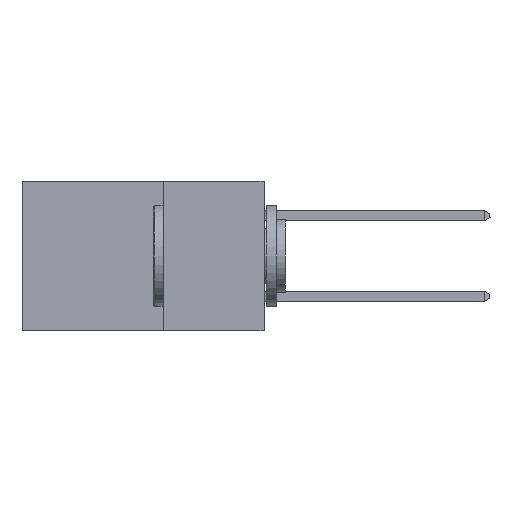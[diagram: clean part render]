
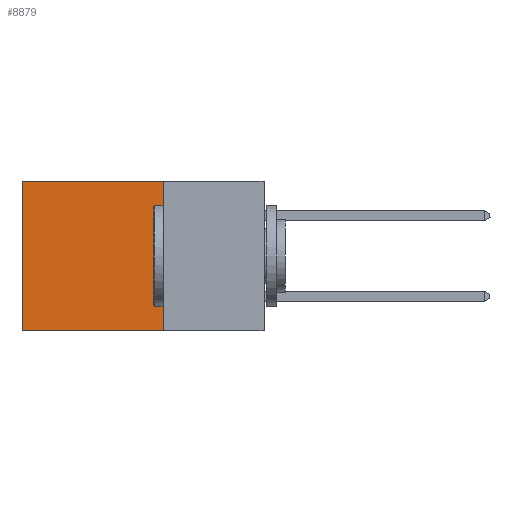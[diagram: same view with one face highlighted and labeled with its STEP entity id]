
A CAD part, left-side view. The second image highlights one B-rep face of the part: STEP entity #8879.
In plain terms, the highlighted planar face has unit normal (-1, 0, 0).
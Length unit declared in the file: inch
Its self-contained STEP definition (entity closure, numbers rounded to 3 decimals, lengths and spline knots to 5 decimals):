
#443 = LINE ( 'NONE', #2643, #15440 ) ;
#2643 = CARTESIAN_POINT ( 'NONE',  ( 0.298, 0.25, 0. ) ) ;
#2981 = CARTESIAN_POINT ( 'NONE',  ( 0.298, 0.25, 0. ) ) ;
#4487 = VERTEX_POINT ( 'NONE', #19841 ) ;
#7111 = AXIS2_PLACEMENT_3D ( 'NONE', #16543, #26297, #11472 ) ;
#8025 = LINE ( 'NONE', #15118, #19415 ) ;
#8879 = ADVANCED_FACE ( 'NONE', ( #30344 ), #21218, .F. ) ;
#10513 = ORIENTED_EDGE ( 'NONE', *, *, #15867, .T. ) ;
#11425 = CARTESIAN_POINT ( 'NONE',  ( 0.298, 0.6, 0. ) ) ;
#11472 = DIRECTION ( 'NONE',  ( 0., 0., -1. ) ) ;
#12732 = DIRECTION ( 'NONE',  ( 0., 0., -1. ) ) ;
#13206 = DIRECTION ( 'NONE',  ( 0., 1., 0. ) ) ;
#14873 = VERTEX_POINT ( 'NONE', #21561 ) ;
#15118 = CARTESIAN_POINT ( 'NONE',  ( 0.298, 0.25, -0.37 ) ) ;
#15440 = VECTOR ( 'NONE', #30175, 39.37008 ) ;
#15867 = EDGE_CURVE ( 'NONE', #4487, #25518, #17449, .T. ) ;
#16543 = CARTESIAN_POINT ( 'NONE',  ( 0.298, 0.25, 0. ) ) ;
#16840 = ORIENTED_EDGE ( 'NONE', *, *, #27438, .T. ) ;
#17449 = LINE ( 'NONE', #11425, #19404 ) ;
#19404 = VECTOR ( 'NONE', #12732, 39.37008 ) ;
#19415 = VECTOR ( 'NONE', #29818, 39.37008 ) ;
#19841 = CARTESIAN_POINT ( 'NONE',  ( 0.298, 0.6, 0. ) ) ;
#20129 = ORIENTED_EDGE ( 'NONE', *, *, #30331, .F. ) ;
#20323 = VECTOR ( 'NONE', #13206, 39.37008 ) ;
#21218 = PLANE ( 'NONE',  #7111 ) ;
#21561 = CARTESIAN_POINT ( 'NONE',  ( 0.298, 0.25, 0. ) ) ;
#22325 = CARTESIAN_POINT ( 'NONE',  ( 0.298, 0.25, -0.37 ) ) ;
#22896 = CARTESIAN_POINT ( 'NONE',  ( 0.298, 0.6, -0.37 ) ) ;
#24707 = ORIENTED_EDGE ( 'NONE', *, *, #28989, .F. ) ;
#25518 = VERTEX_POINT ( 'NONE', #22896 ) ;
#26297 = DIRECTION ( 'NONE',  ( 1., 0., 0. ) ) ;
#26477 = EDGE_LOOP ( 'NONE', ( #10513, #24707, #20129, #16840 ) ) ;
#26702 = VERTEX_POINT ( 'NONE', #22325 ) ;
#27438 = EDGE_CURVE ( 'NONE', #14873, #4487, #31701, .T. ) ;
#28989 = EDGE_CURVE ( 'NONE', #26702, #25518, #8025, .T. ) ;
#29818 = DIRECTION ( 'NONE',  ( 0., 1., 0. ) ) ;
#30175 = DIRECTION ( 'NONE',  ( 0., 0., -1. ) ) ;
#30331 = EDGE_CURVE ( 'NONE', #14873, #26702, #443, .T. ) ;
#30344 = FACE_OUTER_BOUND ( 'NONE', #26477, .T. ) ;
#31701 = LINE ( 'NONE', #2981, #20323 ) ;
